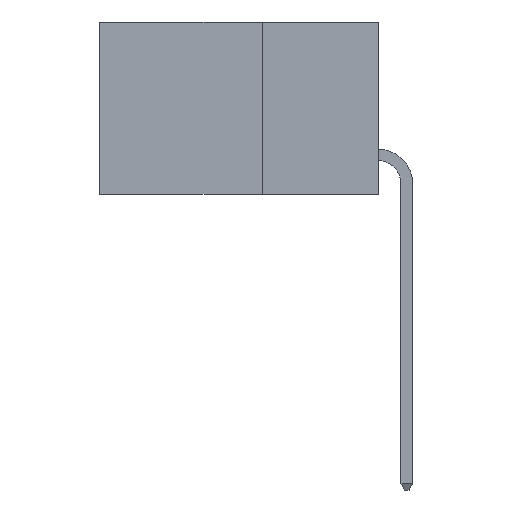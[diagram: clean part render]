
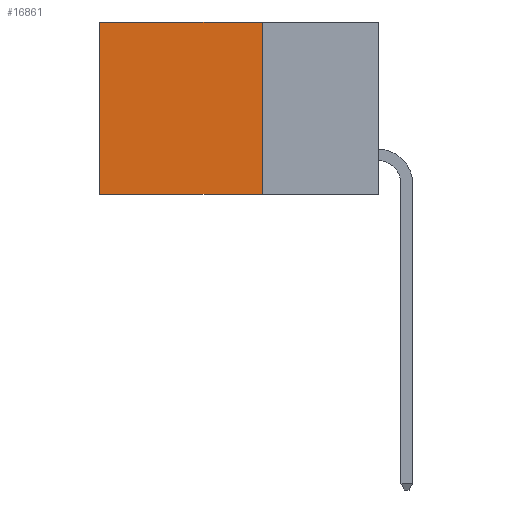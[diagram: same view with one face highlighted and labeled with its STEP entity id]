
A CAD part, left-side view. The second image highlights one B-rep face of the part: STEP entity #16861.
In plain terms, the highlighted planar face has unit normal (-1, 0, 0).
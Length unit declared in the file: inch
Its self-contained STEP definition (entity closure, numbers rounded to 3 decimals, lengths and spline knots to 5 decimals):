
#766 = VERTEX_POINT ( 'NONE', #22460 ) ;
#858 = CARTESIAN_POINT ( 'NONE',  ( 0.2615, 0.6, -0.37 ) ) ;
#931 = DIRECTION ( 'NONE',  ( 1., 0., 0. ) ) ;
#1514 = EDGE_CURVE ( 'NONE', #766, #15725, #20458, .T. ) ;
#1573 = FACE_OUTER_BOUND ( 'NONE', #11925, .T. ) ;
#2552 = ORIENTED_EDGE ( 'NONE', *, *, #5405, .F. ) ;
#2826 = DIRECTION ( 'NONE',  ( 0., 1., 0. ) ) ;
#3443 = ORIENTED_EDGE ( 'NONE', *, *, #21444, .T. ) ;
#3562 = DIRECTION ( 'NONE',  ( 0., 0., -1. ) ) ;
#3933 = VECTOR ( 'NONE', #2826, 39.37008 ) ;
#4491 = PLANE ( 'NONE',  #8452 ) ;
#5405 = EDGE_CURVE ( 'NONE', #15725, #16836, #8624, .T. ) ;
#7627 = DIRECTION ( 'NONE',  ( 0., 0., -1. ) ) ;
#7926 = CARTESIAN_POINT ( 'NONE',  ( 0.2615, 0.25, -0.37 ) ) ;
#8124 = LINE ( 'NONE', #12955, #20326 ) ;
#8452 = AXIS2_PLACEMENT_3D ( 'NONE', #11595, #931, #13373 ) ;
#8624 = LINE ( 'NONE', #11673, #3933 ) ;
#10791 = ORIENTED_EDGE ( 'NONE', *, *, #1514, .F. ) ;
#11586 = EDGE_CURVE ( 'NONE', #12181, #16836, #14619, .T. ) ;
#11595 = CARTESIAN_POINT ( 'NONE',  ( 0.2615, 0.25, -0.37 ) ) ;
#11673 = CARTESIAN_POINT ( 'NONE',  ( 0.2615, 0.25, -0.37 ) ) ;
#11925 = EDGE_LOOP ( 'NONE', ( #22424, #2552, #10791, #3443 ) ) ;
#12020 = CARTESIAN_POINT ( 'NONE',  ( 0.2615, 0.25, -0.37 ) ) ;
#12181 = VERTEX_POINT ( 'NONE', #20840 ) ;
#12955 = CARTESIAN_POINT ( 'NONE',  ( 0.2615, 0.25, 0. ) ) ;
#13373 = DIRECTION ( 'NONE',  ( 0., 0., -1. ) ) ;
#14619 = LINE ( 'NONE', #17583, #22618 ) ;
#15725 = VERTEX_POINT ( 'NONE', #12020 ) ;
#15974 = VECTOR ( 'NONE', #7627, 39.37008 ) ;
#16836 = VERTEX_POINT ( 'NONE', #858 ) ;
#16861 = ADVANCED_FACE ( 'NONE', ( #1573 ), #4491, .F. ) ;
#17583 = CARTESIAN_POINT ( 'NONE',  ( 0.2615, 0.6, -0.37 ) ) ;
#19860 = DIRECTION ( 'NONE',  ( 0., 1., 0. ) ) ;
#20326 = VECTOR ( 'NONE', #19860, 39.37008 ) ;
#20458 = LINE ( 'NONE', #7926, #15974 ) ;
#20840 = CARTESIAN_POINT ( 'NONE',  ( 0.2615, 0.6, 0. ) ) ;
#21444 = EDGE_CURVE ( 'NONE', #766, #12181, #8124, .T. ) ;
#22424 = ORIENTED_EDGE ( 'NONE', *, *, #11586, .T. ) ;
#22460 = CARTESIAN_POINT ( 'NONE',  ( 0.2615, 0.25, 0. ) ) ;
#22618 = VECTOR ( 'NONE', #3562, 39.37008 ) ;
